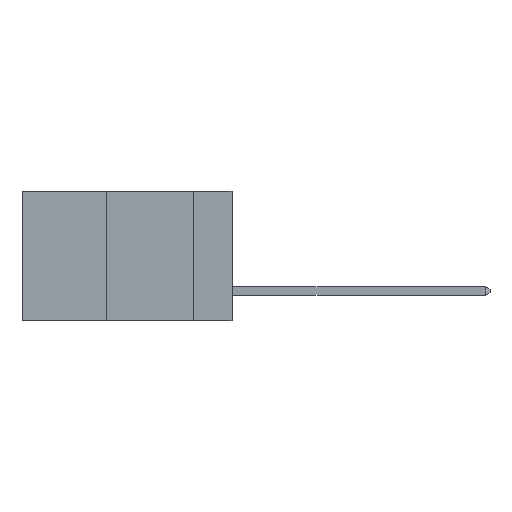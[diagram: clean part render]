
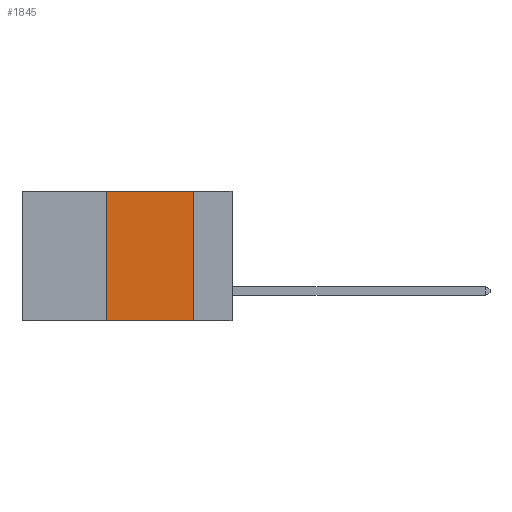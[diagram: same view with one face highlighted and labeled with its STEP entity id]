
A CAD part, left-side view. The second image highlights one B-rep face of the part: STEP entity #1845.
In plain terms, the highlighted planar face has unit normal (-1, 0, 0).
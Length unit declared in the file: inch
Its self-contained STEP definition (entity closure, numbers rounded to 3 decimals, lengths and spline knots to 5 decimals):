
#1810 = VECTOR ( 'NONE', #7996, 39.37008 ) ;
#1845 = ADVANCED_FACE ( 'NONE', ( #13934 ), #11286, .F. ) ;
#1863 = ORIENTED_EDGE ( 'NONE', *, *, #19041, .T. ) ;
#2735 = EDGE_CURVE ( 'NONE', #13910, #9645, #18588, .T. ) ;
#3159 = CARTESIAN_POINT ( 'NONE',  ( 0., 0.36, 0. ) ) ;
#3340 = CARTESIAN_POINT ( 'NONE',  ( 0., 0.11, 0. ) ) ;
#3638 = DIRECTION ( 'NONE',  ( 0., 0., -1. ) ) ;
#5165 = EDGE_CURVE ( 'NONE', #19448, #13910, #12854, .T. ) ;
#6612 = VECTOR ( 'NONE', #10030, 39.37008 ) ;
#7628 = CARTESIAN_POINT ( 'NONE',  ( 0., 0.6, 0. ) ) ;
#7667 = DIRECTION ( 'NONE',  ( 0., -1., 0. ) ) ;
#7996 = DIRECTION ( 'NONE',  ( 0., 0., 1. ) ) ;
#9645 = VERTEX_POINT ( 'NONE', #15589 ) ;
#10030 = DIRECTION ( 'NONE',  ( 0., -1., 0. ) ) ;
#10654 = DIRECTION ( 'NONE',  ( 0., 0., -1. ) ) ;
#10729 = DIRECTION ( 'NONE',  ( 1., 0., 0. ) ) ;
#10820 = CARTESIAN_POINT ( 'NONE',  ( 0., 0.36, -0.37 ) ) ;
#11286 = PLANE ( 'NONE',  #13755 ) ;
#11481 = CARTESIAN_POINT ( 'NONE',  ( 0., 0.6, 0. ) ) ;
#12697 = EDGE_CURVE ( 'NONE', #19922, #19448, #14406, .T. ) ;
#12854 = LINE ( 'NONE', #7628, #16280 ) ;
#13542 = ORIENTED_EDGE ( 'NONE', *, *, #5165, .F. ) ;
#13755 = AXIS2_PLACEMENT_3D ( 'NONE', #11481, #10729, #10654 ) ;
#13910 = VERTEX_POINT ( 'NONE', #17117 ) ;
#13934 = FACE_OUTER_BOUND ( 'NONE', #14936, .T. ) ;
#14107 = CARTESIAN_POINT ( 'NONE',  ( 0., 0.36, 0. ) ) ;
#14406 = LINE ( 'NONE', #3159, #1810 ) ;
#14795 = VECTOR ( 'NONE', #3638, 39.37008 ) ;
#14821 = LINE ( 'NONE', #17506, #6612 ) ;
#14936 = EDGE_LOOP ( 'NONE', ( #16923, #13542, #17372, #1863 ) ) ;
#15589 = CARTESIAN_POINT ( 'NONE',  ( 0., 0.11, -0.37 ) ) ;
#16280 = VECTOR ( 'NONE', #7667, 39.37008 ) ;
#16923 = ORIENTED_EDGE ( 'NONE', *, *, #2735, .F. ) ;
#17117 = CARTESIAN_POINT ( 'NONE',  ( 0., 0.11, 0. ) ) ;
#17372 = ORIENTED_EDGE ( 'NONE', *, *, #12697, .F. ) ;
#17506 = CARTESIAN_POINT ( 'NONE',  ( 0., 0.6, -0.37 ) ) ;
#18588 = LINE ( 'NONE', #3340, #14795 ) ;
#19041 = EDGE_CURVE ( 'NONE', #19922, #9645, #14821, .T. ) ;
#19448 = VERTEX_POINT ( 'NONE', #14107 ) ;
#19922 = VERTEX_POINT ( 'NONE', #10820 ) ;
